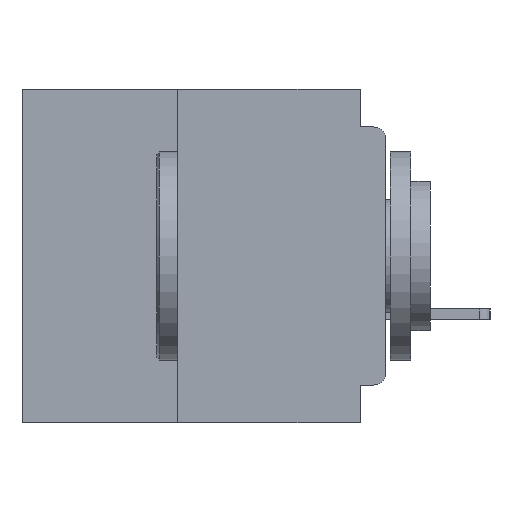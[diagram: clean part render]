
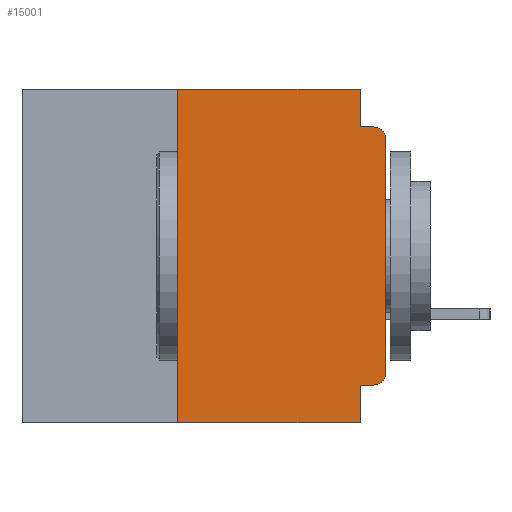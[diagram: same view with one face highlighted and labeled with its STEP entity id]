
A CAD part, left-side view. The second image highlights one B-rep face of the part: STEP entity #15001.
In plain terms, the highlighted planar face has unit normal (-1, 0, 0).
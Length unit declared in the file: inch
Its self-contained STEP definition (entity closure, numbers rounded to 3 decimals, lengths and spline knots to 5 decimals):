
#796 = CARTESIAN_POINT ( 'NONE',  ( 0., 0., -0.045 ) ) ;
#952 = VERTEX_POINT ( 'NONE', #31470 ) ;
#1429 = DIRECTION ( 'NONE',  ( -1., 0., 0. ) ) ;
#1977 = DIRECTION ( 'NONE',  ( -1., 0., 0. ) ) ;
#2931 = VERTEX_POINT ( 'NONE', #13202 ) ;
#6590 = LINE ( 'NONE', #53371, #60947 ) ;
#8497 = CARTESIAN_POINT ( 'NONE',  ( 0., 0.031, -0.4 ) ) ;
#9027 = CARTESIAN_POINT ( 'NONE',  ( 0., 0.031, 0. ) ) ;
#9100 = ORIENTED_EDGE ( 'NONE', *, *, #51649, .F. ) ;
#9691 = VERTEX_POINT ( 'NONE', #43418 ) ;
#9981 = LINE ( 'NONE', #38425, #50355 ) ;
#11450 = CARTESIAN_POINT ( 'NONE',  ( 0., 0.25, -0.4 ) ) ;
#11978 = EDGE_CURVE ( 'NONE', #18623, #34400, #48258, .T. ) ;
#12106 = CARTESIAN_POINT ( 'NONE',  ( 0., 0.437, -0.4 ) ) ;
#13202 = CARTESIAN_POINT ( 'NONE',  ( 0., 0., -0.34 ) ) ;
#14219 = VERTEX_POINT ( 'NONE', #8497 ) ;
#14323 = VERTEX_POINT ( 'NONE', #47185 ) ;
#15001 = ADVANCED_FACE ( 'NONE', ( #36464 ), #37246, .F. ) ;
#15066 = LINE ( 'NONE', #65434, #43065 ) ;
#15194 = AXIS2_PLACEMENT_3D ( 'NONE', #33784, #1977, #39048 ) ;
#15800 = ORIENTED_EDGE ( 'NONE', *, *, #61825, .T. ) ;
#16286 = DIRECTION ( 'NONE',  ( 0., 0., -1. ) ) ;
#16938 = DIRECTION ( 'NONE',  ( 0., -1., 0. ) ) ;
#17247 = DIRECTION ( 'NONE',  ( 0., 1., 0. ) ) ;
#18164 = ORIENTED_EDGE ( 'NONE', *, *, #31740, .T. ) ;
#18623 = VERTEX_POINT ( 'NONE', #19319 ) ;
#18818 = ORIENTED_EDGE ( 'NONE', *, *, #32846, .T. ) ;
#19319 = CARTESIAN_POINT ( 'NONE',  ( 0., 0., -0.06 ) ) ;
#22961 = EDGE_CURVE ( 'NONE', #952, #61033, #32139, .T. ) ;
#23508 = AXIS2_PLACEMENT_3D ( 'NONE', #33260, #1429, #38523 ) ;
#23728 = CIRCLE ( 'NONE', #23508, 0.015 ) ;
#24899 = LINE ( 'NONE', #56158, #64967 ) ;
#25067 = ORIENTED_EDGE ( 'NONE', *, *, #46073, .F. ) ;
#31470 = CARTESIAN_POINT ( 'NONE',  ( 0., 0.25, -0.4 ) ) ;
#31740 = EDGE_CURVE ( 'NONE', #34868, #2931, #23728, .T. ) ;
#31756 = VECTOR ( 'NONE', #54168, 39.37008 ) ;
#31946 = ORIENTED_EDGE ( 'NONE', *, *, #34731, .F. ) ;
#32139 = LINE ( 'NONE', #11450, #35429 ) ;
#32631 = ORIENTED_EDGE ( 'NONE', *, *, #56507, .F. ) ;
#32695 = CARTESIAN_POINT ( 'NONE',  ( 0., 0.031, -0.045 ) ) ;
#32846 = EDGE_CURVE ( 'NONE', #952, #14219, #50617, .T. ) ;
#33260 = CARTESIAN_POINT ( 'NONE',  ( 0., 0.015, -0.34 ) ) ;
#33784 = CARTESIAN_POINT ( 'NONE',  ( 0., 0.015, -0.06 ) ) ;
#34400 = VERTEX_POINT ( 'NONE', #46975 ) ;
#34731 = EDGE_CURVE ( 'NONE', #9691, #14219, #15066, .T. ) ;
#34868 = VERTEX_POINT ( 'NONE', #66557 ) ;
#35429 = VECTOR ( 'NONE', #58969, 39.37008 ) ;
#36464 = FACE_OUTER_BOUND ( 'NONE', #49475, .T. ) ;
#37246 = PLANE ( 'NONE',  #66757 ) ;
#37811 = DIRECTION ( 'NONE',  ( 0., 0., 1. ) ) ;
#38425 = CARTESIAN_POINT ( 'NONE',  ( 0., 0., -0.355 ) ) ;
#38523 = DIRECTION ( 'NONE',  ( 0., 0., -1. ) ) ;
#39048 = DIRECTION ( 'NONE',  ( 0., 0., -1. ) ) ;
#39403 = DIRECTION ( 'NONE',  ( 0., 0., -1. ) ) ;
#40579 = ORIENTED_EDGE ( 'NONE', *, *, #11978, .T. ) ;
#40809 = VECTOR ( 'NONE', #16938, 39.37008 ) ;
#42438 = LINE ( 'NONE', #796, #40809 ) ;
#43065 = VECTOR ( 'NONE', #39403, 39.37008 ) ;
#43301 = VERTEX_POINT ( 'NONE', #32695 ) ;
#43418 = CARTESIAN_POINT ( 'NONE',  ( 0., 0.031, -0.355 ) ) ;
#46073 = EDGE_CURVE ( 'NONE', #14323, #43301, #66647, .T. ) ;
#46975 = CARTESIAN_POINT ( 'NONE',  ( 0., 0.015, -0.045 ) ) ;
#47185 = CARTESIAN_POINT ( 'NONE',  ( 0., 0.031, 0. ) ) ;
#47554 = CARTESIAN_POINT ( 'NONE',  ( 0., 0.437, 0. ) ) ;
#47783 = DIRECTION ( 'NONE',  ( 1., 0., 0. ) ) ;
#48258 = CIRCLE ( 'NONE', #15194, 0.015 ) ;
#49475 = EDGE_LOOP ( 'NONE', ( #15800, #40579, #62804, #25067, #32631, #54416, #18818, #31946, #9100, #18164 ) ) ;
#50355 = VECTOR ( 'NONE', #17247, 39.37008 ) ;
#50617 = LINE ( 'NONE', #12106, #31756 ) ;
#50897 = DIRECTION ( 'NONE',  ( 0., -1., 0. ) ) ;
#51649 = EDGE_CURVE ( 'NONE', #34868, #9691, #9981, .T. ) ;
#52750 = VECTOR ( 'NONE', #56197, 39.37008 ) ;
#53371 = CARTESIAN_POINT ( 'NONE',  ( 0., 0., 0. ) ) ;
#54168 = DIRECTION ( 'NONE',  ( 0., -1., 0. ) ) ;
#54416 = ORIENTED_EDGE ( 'NONE', *, *, #22961, .F. ) ;
#56158 = CARTESIAN_POINT ( 'NONE',  ( 0., 0.437, 0. ) ) ;
#56197 = DIRECTION ( 'NONE',  ( 0., 0., -1. ) ) ;
#56507 = EDGE_CURVE ( 'NONE', #61033, #14323, #24899, .T. ) ;
#58969 = DIRECTION ( 'NONE',  ( 0., 0., 1. ) ) ;
#60947 = VECTOR ( 'NONE', #37811, 39.37008 ) ;
#61033 = VERTEX_POINT ( 'NONE', #67767 ) ;
#61825 = EDGE_CURVE ( 'NONE', #2931, #18623, #6590, .T. ) ;
#62804 = ORIENTED_EDGE ( 'NONE', *, *, #65651, .F. ) ;
#64967 = VECTOR ( 'NONE', #50897, 39.37008 ) ;
#65434 = CARTESIAN_POINT ( 'NONE',  ( 0., 0.031, -0.4 ) ) ;
#65651 = EDGE_CURVE ( 'NONE', #43301, #34400, #42438, .T. ) ;
#66557 = CARTESIAN_POINT ( 'NONE',  ( 0., 0.015, -0.355 ) ) ;
#66647 = LINE ( 'NONE', #9027, #52750 ) ;
#66757 = AXIS2_PLACEMENT_3D ( 'NONE', #47554, #47783, #16286 ) ;
#67767 = CARTESIAN_POINT ( 'NONE',  ( 0., 0.25, 0. ) ) ;
